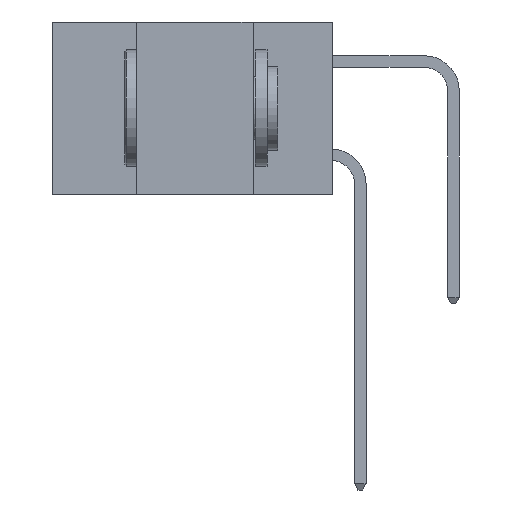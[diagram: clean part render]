
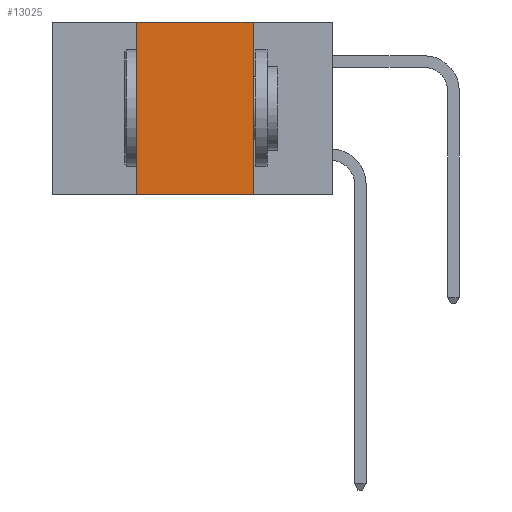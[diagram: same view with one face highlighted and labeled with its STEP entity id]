
A CAD part, left-side view. The second image highlights one B-rep face of the part: STEP entity #13025.
In plain terms, the highlighted planar face has unit normal (-1, 0, 0).
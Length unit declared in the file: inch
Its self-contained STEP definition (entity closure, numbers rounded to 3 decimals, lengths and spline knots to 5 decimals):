
#138 = FACE_OUTER_BOUND ( 'NONE', #9887, .T. ) ;
#690 = VECTOR ( 'NONE', #14820, 39.37008 ) ;
#1321 = DIRECTION ( 'NONE',  ( 0., 0., -1. ) ) ;
#1726 = ORIENTED_EDGE ( 'NONE', *, *, #14601, .F. ) ;
#1905 = LINE ( 'NONE', #17523, #12853 ) ;
#3580 = CARTESIAN_POINT ( 'NONE',  ( 0., 0.42, 0. ) ) ;
#4670 = LINE ( 'NONE', #13716, #26587 ) ;
#7813 = CARTESIAN_POINT ( 'NONE',  ( 0., 0.42, -0.37 ) ) ;
#7819 = AXIS2_PLACEMENT_3D ( 'NONE', #26824, #14347, #1321 ) ;
#8178 = ORIENTED_EDGE ( 'NONE', *, *, #20939, .F. ) ;
#8811 = VECTOR ( 'NONE', #12906, 39.37008 ) ;
#9887 = EDGE_LOOP ( 'NONE', ( #23804, #1726, #8178, #14013 ) ) ;
#11369 = EDGE_CURVE ( 'NONE', #15489, #21113, #1905, .T. ) ;
#12695 = CARTESIAN_POINT ( 'NONE',  ( 0., 0.6, 0. ) ) ;
#12853 = VECTOR ( 'NONE', #19579, 39.37008 ) ;
#12906 = DIRECTION ( 'NONE',  ( 0., -1., 0. ) ) ;
#13025 = ADVANCED_FACE ( 'NONE', ( #138 ), #16378, .F. ) ;
#13716 = CARTESIAN_POINT ( 'NONE',  ( 0., 0.42, -0.37 ) ) ;
#14013 = ORIENTED_EDGE ( 'NONE', *, *, #20049, .T. ) ;
#14347 = DIRECTION ( 'NONE',  ( 1., 0., 0. ) ) ;
#14601 = EDGE_CURVE ( 'NONE', #17481, #15489, #17915, .T. ) ;
#14820 = DIRECTION ( 'NONE',  ( 0., -1., 0. ) ) ;
#15489 = VERTEX_POINT ( 'NONE', #25720 ) ;
#15854 = VERTEX_POINT ( 'NONE', #7813 ) ;
#16378 = PLANE ( 'NONE',  #7819 ) ;
#17481 = VERTEX_POINT ( 'NONE', #3580 ) ;
#17523 = CARTESIAN_POINT ( 'NONE',  ( 0., 0.17, -0.37 ) ) ;
#17915 = LINE ( 'NONE', #12695, #690 ) ;
#19579 = DIRECTION ( 'NONE',  ( 0., 0., -1. ) ) ;
#20011 = DIRECTION ( 'NONE',  ( 0., 0., 1. ) ) ;
#20049 = EDGE_CURVE ( 'NONE', #15854, #21113, #20797, .T. ) ;
#20458 = CARTESIAN_POINT ( 'NONE',  ( 0., 0.17, -0.37 ) ) ;
#20797 = LINE ( 'NONE', #23330, #8811 ) ;
#20939 = EDGE_CURVE ( 'NONE', #15854, #17481, #4670, .T. ) ;
#21113 = VERTEX_POINT ( 'NONE', #20458 ) ;
#23330 = CARTESIAN_POINT ( 'NONE',  ( 0., 0.6, -0.37 ) ) ;
#23804 = ORIENTED_EDGE ( 'NONE', *, *, #11369, .F. ) ;
#25720 = CARTESIAN_POINT ( 'NONE',  ( 0., 0.17, 0. ) ) ;
#26587 = VECTOR ( 'NONE', #20011, 39.37008 ) ;
#26824 = CARTESIAN_POINT ( 'NONE',  ( 0., 0.6, 0. ) ) ;
